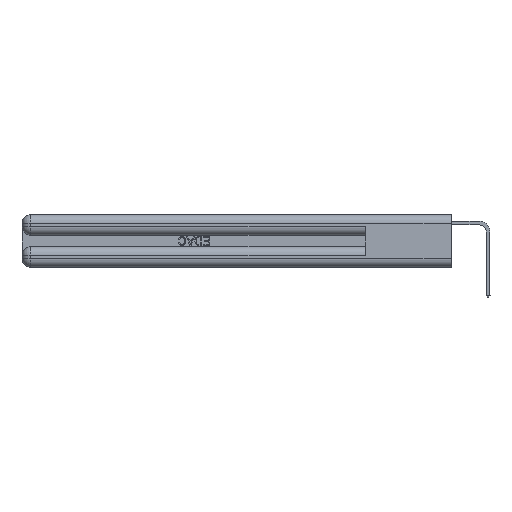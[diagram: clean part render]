
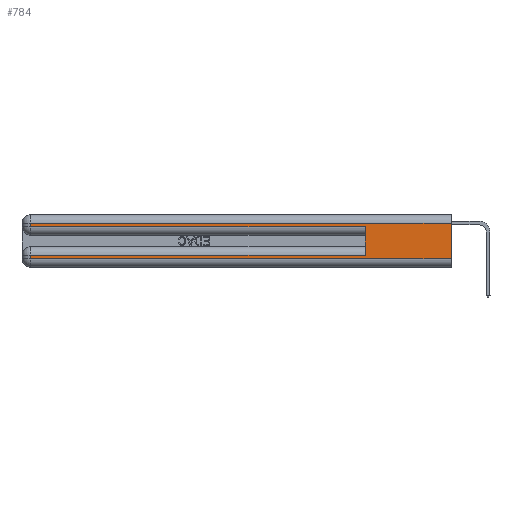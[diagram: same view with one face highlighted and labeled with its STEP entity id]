
A CAD part, left-side view. The second image highlights one B-rep face of the part: STEP entity #784.
In plain terms, the highlighted planar face has unit normal (-1, 0, 0).
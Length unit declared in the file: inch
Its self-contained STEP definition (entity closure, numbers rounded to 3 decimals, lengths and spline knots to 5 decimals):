
#120 = VERTEX_POINT ( 'NONE', #21641 ) ;
#252 = DIRECTION ( 'NONE',  ( 0., -1., 0. ) ) ;
#641 = CARTESIAN_POINT ( 'NONE',  ( 0., 2.94, 0.085 ) ) ;
#784 = ADVANCED_FACE ( 'NONE', ( #30864 ), #18286, .F. ) ;
#938 = LINE ( 'NONE', #20831, #19127 ) ;
#1009 = VERTEX_POINT ( 'NONE', #641 ) ;
#1171 = VERTEX_POINT ( 'NONE', #13525 ) ;
#3564 = EDGE_LOOP ( 'NONE', ( #18437, #27740, #30954, #5027, #15431, #10276, #31534, #30108 ) ) ;
#3698 = VECTOR ( 'NONE', #14371, 39.37008 ) ;
#3855 = LINE ( 'NONE', #23897, #9228 ) ;
#4100 = DIRECTION ( 'NONE',  ( 1., 0., 0. ) ) ;
#4322 = EDGE_CURVE ( 'NONE', #15936, #120, #11724, .T. ) ;
#4558 = EDGE_CURVE ( 'NONE', #15747, #1009, #938, .T. ) ;
#4950 = EDGE_CURVE ( 'NONE', #1171, #20773, #32084, .T. ) ;
#5027 = ORIENTED_EDGE ( 'NONE', *, *, #4950, .T. ) ;
#5699 = DIRECTION ( 'NONE',  ( 0., 0., -1. ) ) ;
#6702 = EDGE_CURVE ( 'NONE', #15936, #31336, #15871, .T. ) ;
#6879 = LINE ( 'NONE', #16827, #3698 ) ;
#7002 = DIRECTION ( 'NONE',  ( 0., 0., -1. ) ) ;
#7055 = VECTOR ( 'NONE', #18149, 39.37008 ) ;
#8454 = CARTESIAN_POINT ( 'NONE',  ( 0., 2.94, 0.37 ) ) ;
#8629 = CARTESIAN_POINT ( 'NONE',  ( 0., 2.94, 0.06 ) ) ;
#8724 = DIRECTION ( 'NONE',  ( 0., -1., 0. ) ) ;
#9228 = VECTOR ( 'NONE', #31912, 39.37008 ) ;
#9458 = CARTESIAN_POINT ( 'NONE',  ( 0., 0., 0.37 ) ) ;
#10276 = ORIENTED_EDGE ( 'NONE', *, *, #4558, .T. ) ;
#11318 = CARTESIAN_POINT ( 'NONE',  ( 0., 0., 0.31 ) ) ;
#11460 = VECTOR ( 'NONE', #7002, 39.37008 ) ;
#11724 = LINE ( 'NONE', #9458, #11460 ) ;
#13336 = VECTOR ( 'NONE', #252, 39.37008 ) ;
#13525 = CARTESIAN_POINT ( 'NONE',  ( 0., 2.94, 0.285 ) ) ;
#14371 = DIRECTION ( 'NONE',  ( 0., 0., 1. ) ) ;
#14702 = EDGE_CURVE ( 'NONE', #15747, #20773, #6879, .T. ) ;
#15181 = VECTOR ( 'NONE', #5699, 39.37008 ) ;
#15431 = ORIENTED_EDGE ( 'NONE', *, *, #14702, .F. ) ;
#15747 = VERTEX_POINT ( 'NONE', #25368 ) ;
#15871 = LINE ( 'NONE', #30565, #7055 ) ;
#15936 = VERTEX_POINT ( 'NONE', #11318 ) ;
#16336 = DIRECTION ( 'NONE',  ( 0., 0., -1. ) ) ;
#16827 = CARTESIAN_POINT ( 'NONE',  ( 0., 0.6, 0.145 ) ) ;
#17626 = CARTESIAN_POINT ( 'NONE',  ( 0., 0.6, 0.285 ) ) ;
#17729 = VECTOR ( 'NONE', #8724, 39.37008 ) ;
#18149 = DIRECTION ( 'NONE',  ( 0., 1., 0. ) ) ;
#18286 = PLANE ( 'NONE',  #26836 ) ;
#18437 = ORIENTED_EDGE ( 'NONE', *, *, #4322, .F. ) ;
#18984 = CARTESIAN_POINT ( 'NONE',  ( 0., 0., 0.06 ) ) ;
#19032 = CARTESIAN_POINT ( 'NONE',  ( 0., 2.94, 0.31 ) ) ;
#19127 = VECTOR ( 'NONE', #25738, 39.37008 ) ;
#20773 = VERTEX_POINT ( 'NONE', #17626 ) ;
#20831 = CARTESIAN_POINT ( 'NONE',  ( 0., 0., 0.085 ) ) ;
#21592 = LINE ( 'NONE', #18984, #17729 ) ;
#21641 = CARTESIAN_POINT ( 'NONE',  ( 0., 0., 0.06 ) ) ;
#22594 = CARTESIAN_POINT ( 'NONE',  ( 0., 0., 0.285 ) ) ;
#23104 = EDGE_CURVE ( 'NONE', #29517, #120, #21592, .T. ) ;
#23330 = CARTESIAN_POINT ( 'NONE',  ( 0., 0., 0.37 ) ) ;
#23897 = CARTESIAN_POINT ( 'NONE',  ( 0., 2.94, 0.37 ) ) ;
#24395 = EDGE_CURVE ( 'NONE', #31336, #1171, #30967, .T. ) ;
#25368 = CARTESIAN_POINT ( 'NONE',  ( 0., 0.6, 0.085 ) ) ;
#25738 = DIRECTION ( 'NONE',  ( 0., 1., 0. ) ) ;
#26836 = AXIS2_PLACEMENT_3D ( 'NONE', #23330, #4100, #16336 ) ;
#27740 = ORIENTED_EDGE ( 'NONE', *, *, #6702, .T. ) ;
#29517 = VERTEX_POINT ( 'NONE', #8629 ) ;
#30108 = ORIENTED_EDGE ( 'NONE', *, *, #23104, .T. ) ;
#30565 = CARTESIAN_POINT ( 'NONE',  ( 0., 0., 0.31 ) ) ;
#30864 = FACE_OUTER_BOUND ( 'NONE', #3564, .T. ) ;
#30954 = ORIENTED_EDGE ( 'NONE', *, *, #24395, .T. ) ;
#30967 = LINE ( 'NONE', #8454, #15181 ) ;
#31336 = VERTEX_POINT ( 'NONE', #19032 ) ;
#31534 = ORIENTED_EDGE ( 'NONE', *, *, #31653, .T. ) ;
#31653 = EDGE_CURVE ( 'NONE', #1009, #29517, #3855, .T. ) ;
#31912 = DIRECTION ( 'NONE',  ( 0., 0., -1. ) ) ;
#32084 = LINE ( 'NONE', #22594, #13336 ) ;
